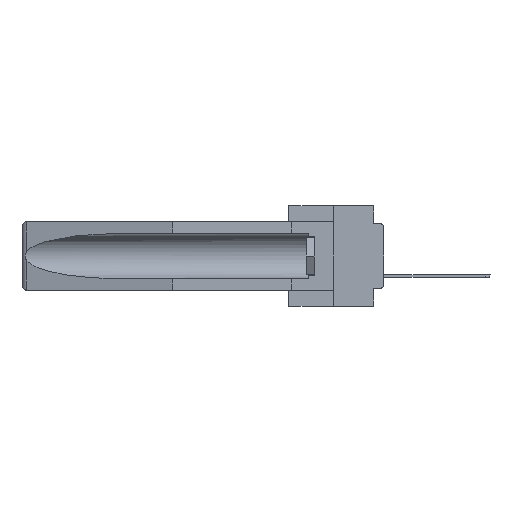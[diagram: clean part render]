
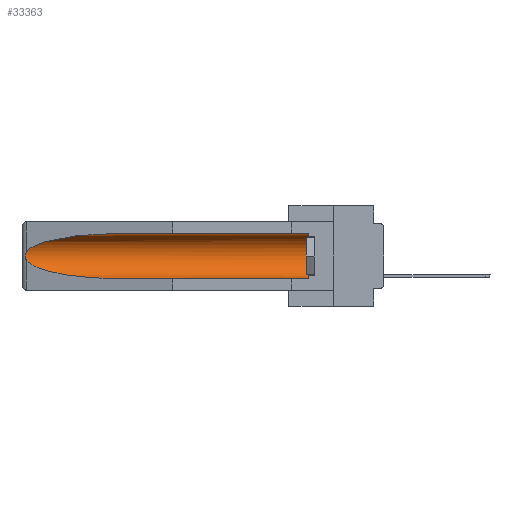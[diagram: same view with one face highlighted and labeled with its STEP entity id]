
A CAD part, left-side view. The second image highlights one B-rep face of the part: STEP entity #33363.
In plain terms, the highlighted cylindrical face has radius 2.857 mm (diameter 5.715 mm), a partial arc.
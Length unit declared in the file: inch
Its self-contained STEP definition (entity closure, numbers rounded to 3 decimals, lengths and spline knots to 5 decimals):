
#120 = CARTESIAN_POINT ( 'NONE',  ( 0.26597, 1.52961, -0.15275 ) ) ;
#723 = VERTEX_POINT ( 'NONE', #26273 ) ;
#1097 = CYLINDRICAL_SURFACE ( 'NONE', #5018, 0.1125 ) ;
#1117 = CARTESIAN_POINT ( 'NONE',  ( 0.21114, 1.30732, -0.284 ) ) ;
#1814 = EDGE_CURVE ( 'NONE', #3810, #22496, #23741, .T. ) ;
#2033 = CARTESIAN_POINT ( 'NONE',  ( 0.26597, 1.5296, -0.19026 ) ) ;
#2090 = ORIENTED_EDGE ( 'NONE', *, *, #23298, .T. ) ;
#2184 = CARTESIAN_POINT ( 'NONE',  ( 0.2675, 1.53308, -0.16763 ) ) ;
#2692 = CARTESIAN_POINT ( 'NONE',  ( 0.155, 1.07973, -0.284 ) ) ;
#2998 = VECTOR ( 'NONE', #18564, 39.37008 ) ;
#3425 = CARTESIAN_POINT ( 'NONE',  ( 0.155, 0.126, -0.1715 ) ) ;
#3810 = VERTEX_POINT ( 'NONE', #9891 ) ;
#5018 = AXIS2_PLACEMENT_3D ( 'NONE', #8993, #30021, #24841 ) ;
#5435 = CARTESIAN_POINT ( 'NONE',  ( 0.2673, 1.5327, -0.16383 ) ) ;
#6841 = ORIENTED_EDGE ( 'NONE', *, *, #26160, .T. ) ;
#6969 = CARTESIAN_POINT ( 'NONE',  ( 0.25451, 1.48313, -0.09465 ) ) ;
#7207 = DIRECTION ( 'NONE',  ( 0., 1., 0. ) ) ;
#7665 = CARTESIAN_POINT ( 'NONE',  ( 0.26537, 1.52718, -0.19328 ) ) ;
#8993 = CARTESIAN_POINT ( 'NONE',  ( 0.155, -0.30754, -0.1715 ) ) ;
#9175 = CARTESIAN_POINT ( 'NONE',  ( 0.26537, 1.52718, -0.19328 ) ) ;
#9236 = VERTEX_POINT ( 'NONE', #9491 ) ;
#9491 = CARTESIAN_POINT ( 'NONE',  ( 0.26537, 1.52718, -0.19328 ) ) ;
#9876 = VERTEX_POINT ( 'NONE', #24724 ) ;
#9891 = CARTESIAN_POINT ( 'NONE',  ( 0.155, 0.126, -0.284 ) ) ;
#10253 = CARTESIAN_POINT ( 'NONE',  ( 0.26537, 1.52718, -0.14972 ) ) ;
#11482 = ORIENTED_EDGE ( 'NONE', *, *, #18172, .T. ) ;
#11581 = CARTESIAN_POINT ( 'NONE',  ( 0.155, 1.07973, -0.284 ) ) ;
#11646 = DIRECTION ( 'NONE',  ( 0., 0., 1. ) ) ;
#12394 = CARTESIAN_POINT ( 'NONE',  ( 0.155, -0.30754, -0.059 ) ) ;
#16487 = DIRECTION ( 'NONE',  ( 0., -1., 0. ) ) ;
#16953 = CARTESIAN_POINT ( 'NONE',  ( 0.155, 1.07973, -0.059 ) ) ;
#17129 = EDGE_CURVE ( 'NONE', #3810, #723, #30322, .T. ) ;
#17268 = B_SPLINE_CURVE_WITH_KNOTS ( 'NONE', 3,
 ( #10253, #120, #18166, #5435, #2184, #23164, #25600, #31435, #2033, #7665 ),
 .UNSPECIFIED., .F., .F.,
 ( 4, 2, 2, 2, 4 ),
 ( 0., 0.00029, 0.00058, 0.00087, 0.00117 ),
 .UNSPECIFIED. ) ;
#18166 = CARTESIAN_POINT ( 'NONE',  ( 0.26654, 1.53092, -0.15636 ) ) ;
#18172 = EDGE_CURVE ( 'NONE', #723, #29639, #33580, .T. ) ;
#18421 =( BOUNDED_CURVE ( )  B_SPLINE_CURVE ( 3, ( #22322, #22828, #6969, #32817 ),
 .UNSPECIFIED., .F., .T. ) 
 B_SPLINE_CURVE_WITH_KNOTS ( ( 4, 4 ),
 ( 4.71239, 6.08839 ),
 .UNSPECIFIED. ) 
 CURVE ( )  GEOMETRIC_REPRESENTATION_ITEM ( )  RATIONAL_B_SPLINE_CURVE ( ( 1., 0.848, 0.848, 1. ) ) 
 REPRESENTATION_ITEM ( '' )  );
#18564 = DIRECTION ( 'NONE',  ( 0., 1., 0. ) ) ;
#19168 = ORIENTED_EDGE ( 'NONE', *, *, #1814, .F. ) ;
#19314 = EDGE_CURVE ( 'NONE', #29639, #9876, #18421, .T. ) ;
#20494 = ORIENTED_EDGE ( 'NONE', *, *, #17129, .T. ) ;
#22322 = CARTESIAN_POINT ( 'NONE',  ( 0.155, 1.07973, -0.059 ) ) ;
#22496 = VERTEX_POINT ( 'NONE', #2692 ) ;
#22828 = CARTESIAN_POINT ( 'NONE',  ( 0.21114, 1.30732, -0.059 ) ) ;
#23164 = CARTESIAN_POINT ( 'NONE',  ( 0.2675, 1.53308, -0.17534 ) ) ;
#23298 = EDGE_CURVE ( 'NONE', #9236, #22496, #30493, .T. ) ;
#23741 = LINE ( 'NONE', #25984, #2998 ) ;
#24724 = CARTESIAN_POINT ( 'NONE',  ( 0.26537, 1.52718, -0.14972 ) ) ;
#24841 = DIRECTION ( 'NONE',  ( 0., 0., 1. ) ) ;
#25600 = CARTESIAN_POINT ( 'NONE',  ( 0.2673, 1.53269, -0.17917 ) ) ;
#25906 = ORIENTED_EDGE ( 'NONE', *, *, #19314, .T. ) ;
#25984 = CARTESIAN_POINT ( 'NONE',  ( 0.155, -0.30754, -0.284 ) ) ;
#26160 = EDGE_CURVE ( 'NONE', #9876, #9236, #17268, .T. ) ;
#26273 = CARTESIAN_POINT ( 'NONE',  ( 0.155, 0.126, -0.059 ) ) ;
#27084 = FACE_OUTER_BOUND ( 'NONE', #30510, .T. ) ;
#28139 = AXIS2_PLACEMENT_3D ( 'NONE', #3425, #16487, #11646 ) ;
#29639 = VERTEX_POINT ( 'NONE', #16953 ) ;
#30021 = DIRECTION ( 'NONE',  ( 0., 1., 0. ) ) ;
#30038 = CARTESIAN_POINT ( 'NONE',  ( 0.25451, 1.48313, -0.24835 ) ) ;
#30322 = CIRCLE ( 'NONE', #28139, 0.1125 ) ;
#30493 =( BOUNDED_CURVE ( )  B_SPLINE_CURVE ( 3, ( #9175, #30038, #1117, #11581 ),
 .UNSPECIFIED., .F., .T. ) 
 B_SPLINE_CURVE_WITH_KNOTS ( ( 4, 4 ),
 ( 0.1948, 1.5708 ),
 .UNSPECIFIED. ) 
 CURVE ( )  GEOMETRIC_REPRESENTATION_ITEM ( )  RATIONAL_B_SPLINE_CURVE ( ( 1., 0.848, 0.848, 1. ) ) 
 REPRESENTATION_ITEM ( '' )  );
#30510 = EDGE_LOOP ( 'NONE', ( #25906, #6841, #2090, #19168, #20494, #11482 ) ) ;
#31435 = CARTESIAN_POINT ( 'NONE',  ( 0.26655, 1.53094, -0.18657 ) ) ;
#31495 = VECTOR ( 'NONE', #7207, 39.37008 ) ;
#32817 = CARTESIAN_POINT ( 'NONE',  ( 0.26537, 1.52718, -0.14972 ) ) ;
#33363 = ADVANCED_FACE ( 'NONE', ( #27084 ), #1097, .F. ) ;
#33580 = LINE ( 'NONE', #12394, #31495 ) ;
